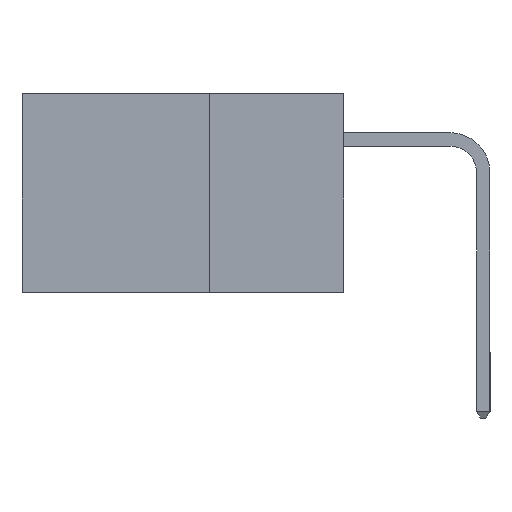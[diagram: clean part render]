
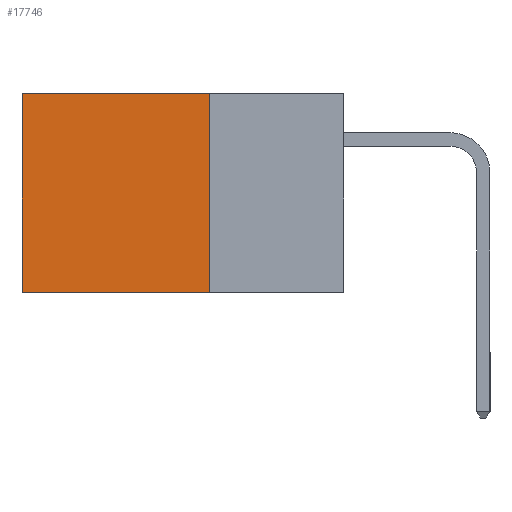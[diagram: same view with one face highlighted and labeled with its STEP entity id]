
A CAD part, left-side view. The second image highlights one B-rep face of the part: STEP entity #17746.
In plain terms, the highlighted planar face has unit normal (-1, 0, 0).
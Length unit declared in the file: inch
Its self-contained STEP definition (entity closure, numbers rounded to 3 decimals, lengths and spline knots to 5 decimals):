
#1264 = DIRECTION ( 'NONE',  ( 0., 0., -1. ) ) ;
#1610 = ORIENTED_EDGE ( 'NONE', *, *, #12775, .F. ) ;
#2961 = CARTESIAN_POINT ( 'NONE',  ( 0.298, 0.25, -0.37 ) ) ;
#3077 = CARTESIAN_POINT ( 'NONE',  ( 0.298, 0.6, -0.37 ) ) ;
#3814 = VECTOR ( 'NONE', #16188, 39.37008 ) ;
#5243 = CARTESIAN_POINT ( 'NONE',  ( 0.298, 0.25, 0. ) ) ;
#6400 = VERTEX_POINT ( 'NONE', #12325 ) ;
#6646 = AXIS2_PLACEMENT_3D ( 'NONE', #5243, #14701, #1264 ) ;
#6752 = EDGE_LOOP ( 'NONE', ( #16086, #1610, #10212, #17084 ) ) ;
#9514 = VECTOR ( 'NONE', #11649, 39.37008 ) ;
#10212 = ORIENTED_EDGE ( 'NONE', *, *, #12853, .F. ) ;
#10862 = FACE_OUTER_BOUND ( 'NONE', #6752, .T. ) ;
#11057 = CARTESIAN_POINT ( 'NONE',  ( 0.298, 0.6, 0. ) ) ;
#11630 = VERTEX_POINT ( 'NONE', #14904 ) ;
#11649 = DIRECTION ( 'NONE',  ( 0., 1., 0. ) ) ;
#12325 = CARTESIAN_POINT ( 'NONE',  ( 0.298, 0.25, 0. ) ) ;
#12775 = EDGE_CURVE ( 'NONE', #16135, #24498, #16299, .T. ) ;
#12853 = EDGE_CURVE ( 'NONE', #6400, #16135, #21738, .T. ) ;
#13687 = CARTESIAN_POINT ( 'NONE',  ( 0.298, 0.25, 0. ) ) ;
#14247 = CARTESIAN_POINT ( 'NONE',  ( 0.298, 0.25, 0. ) ) ;
#14701 = DIRECTION ( 'NONE',  ( 1., 0., 0. ) ) ;
#14801 = EDGE_CURVE ( 'NONE', #6400, #11630, #23459, .T. ) ;
#14904 = CARTESIAN_POINT ( 'NONE',  ( 0.298, 0.6, 0. ) ) ;
#16086 = ORIENTED_EDGE ( 'NONE', *, *, #25156, .T. ) ;
#16135 = VERTEX_POINT ( 'NONE', #2961 ) ;
#16188 = DIRECTION ( 'NONE',  ( 0., 1., 0. ) ) ;
#16299 = LINE ( 'NONE', #18015, #3814 ) ;
#16447 = DIRECTION ( 'NONE',  ( 0., 0., -1. ) ) ;
#17084 = ORIENTED_EDGE ( 'NONE', *, *, #14801, .T. ) ;
#17681 = VECTOR ( 'NONE', #22885, 39.37008 ) ;
#17746 = ADVANCED_FACE ( 'NONE', ( #10862 ), #24591, .F. ) ;
#18015 = CARTESIAN_POINT ( 'NONE',  ( 0.298, 0.25, -0.37 ) ) ;
#20138 = LINE ( 'NONE', #11057, #17681 ) ;
#21409 = VECTOR ( 'NONE', #16447, 39.37008 ) ;
#21738 = LINE ( 'NONE', #14247, #21409 ) ;
#22885 = DIRECTION ( 'NONE',  ( 0., 0., -1. ) ) ;
#23459 = LINE ( 'NONE', #13687, #9514 ) ;
#24498 = VERTEX_POINT ( 'NONE', #3077 ) ;
#24591 = PLANE ( 'NONE',  #6646 ) ;
#25156 = EDGE_CURVE ( 'NONE', #11630, #24498, #20138, .T. ) ;
